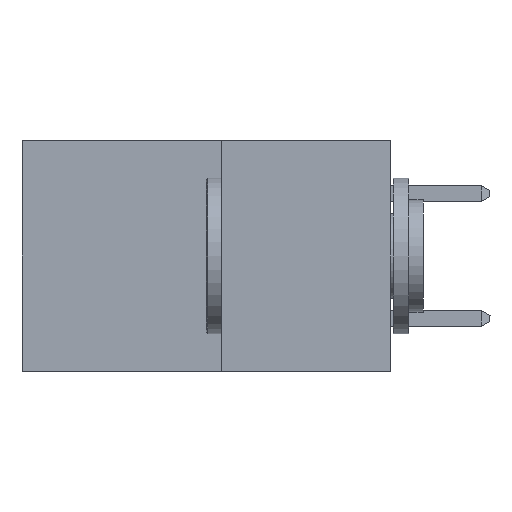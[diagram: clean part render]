
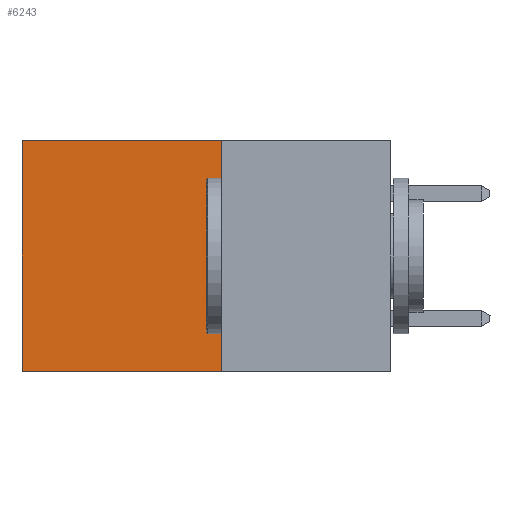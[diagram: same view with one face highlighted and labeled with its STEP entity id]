
A CAD part, left-side view. The second image highlights one B-rep face of the part: STEP entity #6243.
In plain terms, the highlighted planar face has unit normal (-1, 0, 0).
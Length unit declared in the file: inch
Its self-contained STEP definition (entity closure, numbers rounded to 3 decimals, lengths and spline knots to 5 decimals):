
#89 = CARTESIAN_POINT ( 'NONE',  ( 0.277, 0.59, -0.37 ) ) ;
#189 = CARTESIAN_POINT ( 'NONE',  ( 0.277, 0.27, -0.37 ) ) ;
#422 = CARTESIAN_POINT ( 'NONE',  ( 0.277, 0.27, -0.37 ) ) ;
#1162 = CARTESIAN_POINT ( 'NONE',  ( 0.277, 0.59, -0.37 ) ) ;
#1273 = LINE ( 'NONE', #8207, #4946 ) ;
#1542 = VECTOR ( 'NONE', #6455, 39.37008 ) ;
#1562 = VECTOR ( 'NONE', #7508, 39.37008 ) ;
#2119 = VERTEX_POINT ( 'NONE', #2737 ) ;
#2202 = EDGE_CURVE ( 'NONE', #2119, #7213, #7082, .T. ) ;
#2414 = FACE_OUTER_BOUND ( 'NONE', #5496, .T. ) ;
#2737 = CARTESIAN_POINT ( 'NONE',  ( 0.277, 0.27, 0. ) ) ;
#2766 = ORIENTED_EDGE ( 'NONE', *, *, #3196, .T. ) ;
#2954 = DIRECTION ( 'NONE',  ( 0., 0., -1. ) ) ;
#2991 = ORIENTED_EDGE ( 'NONE', *, *, #2202, .F. ) ;
#3196 = EDGE_CURVE ( 'NONE', #4964, #5539, #8511, .T. ) ;
#3735 = EDGE_CURVE ( 'NONE', #7213, #5539, #5848, .T. ) ;
#4365 = DIRECTION ( 'NONE',  ( 0., 1., 0. ) ) ;
#4773 = DIRECTION ( 'NONE',  ( 0., 1., 0. ) ) ;
#4820 = ORIENTED_EDGE ( 'NONE', *, *, #5579, .T. ) ;
#4830 = AXIS2_PLACEMENT_3D ( 'NONE', #189, #7096, #2954 ) ;
#4946 = VECTOR ( 'NONE', #4365, 39.37008 ) ;
#4964 = VERTEX_POINT ( 'NONE', #8039 ) ;
#5496 = EDGE_LOOP ( 'NONE', ( #2766, #6549, #2991, #4820 ) ) ;
#5539 = VERTEX_POINT ( 'NONE', #89 ) ;
#5579 = EDGE_CURVE ( 'NONE', #2119, #4964, #1273, .T. ) ;
#5809 = PLANE ( 'NONE',  #4830 ) ;
#5848 = LINE ( 'NONE', #6183, #8562 ) ;
#6183 = CARTESIAN_POINT ( 'NONE',  ( 0.277, 0.27, -0.37 ) ) ;
#6243 = ADVANCED_FACE ( 'NONE', ( #2414 ), #5809, .F. ) ;
#6455 = DIRECTION ( 'NONE',  ( 0., 0., -1. ) ) ;
#6549 = ORIENTED_EDGE ( 'NONE', *, *, #3735, .F. ) ;
#7082 = LINE ( 'NONE', #8212, #1562 ) ;
#7096 = DIRECTION ( 'NONE',  ( 1., 0., 0. ) ) ;
#7213 = VERTEX_POINT ( 'NONE', #422 ) ;
#7508 = DIRECTION ( 'NONE',  ( 0., 0., -1. ) ) ;
#8039 = CARTESIAN_POINT ( 'NONE',  ( 0.277, 0.59, 0. ) ) ;
#8207 = CARTESIAN_POINT ( 'NONE',  ( 0.277, 0.27, 0. ) ) ;
#8212 = CARTESIAN_POINT ( 'NONE',  ( 0.277, 0.27, -0.37 ) ) ;
#8511 = LINE ( 'NONE', #1162, #1542 ) ;
#8562 = VECTOR ( 'NONE', #4773, 39.37008 ) ;
